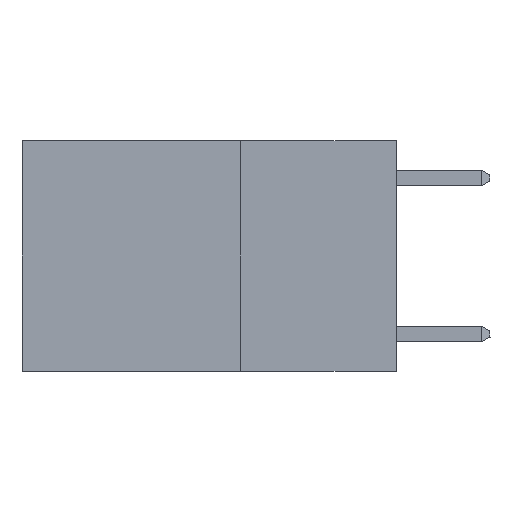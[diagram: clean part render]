
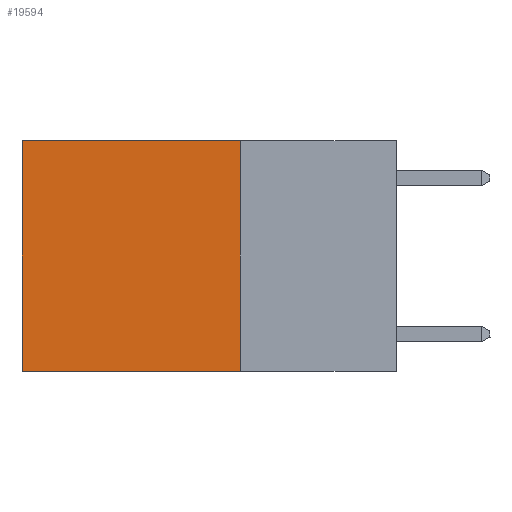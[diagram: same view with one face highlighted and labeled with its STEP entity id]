
A CAD part, left-side view. The second image highlights one B-rep face of the part: STEP entity #19594.
In plain terms, the highlighted planar face has unit normal (-1, 0, 0).
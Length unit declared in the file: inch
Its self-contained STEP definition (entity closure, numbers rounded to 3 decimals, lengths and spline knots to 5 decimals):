
#180 = LINE ( 'NONE', #2613, #320 ) ;
#320 = VECTOR ( 'NONE', #13146, 39.37008 ) ;
#630 = VECTOR ( 'NONE', #18953, 39.37008 ) ;
#824 = LINE ( 'NONE', #12103, #630 ) ;
#914 = ORIENTED_EDGE ( 'NONE', *, *, #18890, .T. ) ;
#1774 = DIRECTION ( 'NONE',  ( 0., 0., -1. ) ) ;
#2613 = CARTESIAN_POINT ( 'NONE',  ( 0.2625, 0.25, 0. ) ) ;
#7074 = CARTESIAN_POINT ( 'NONE',  ( 0.2625, 0.6, 0. ) ) ;
#7731 = EDGE_LOOP ( 'NONE', ( #914, #15957, #12379, #12878 ) ) ;
#8198 = LINE ( 'NONE', #22268, #21597 ) ;
#8571 = CARTESIAN_POINT ( 'NONE',  ( 0.2625, 0.6, 0. ) ) ;
#8824 = DIRECTION ( 'NONE',  ( 0., 0., -1. ) ) ;
#8877 = CARTESIAN_POINT ( 'NONE',  ( 0.2625, 0.25, 0. ) ) ;
#9751 = EDGE_CURVE ( 'NONE', #20449, #17550, #824, .T. ) ;
#10504 = VECTOR ( 'NONE', #8824, 39.37008 ) ;
#10688 = EDGE_CURVE ( 'NONE', #13894, #20034, #180, .T. ) ;
#11238 = CARTESIAN_POINT ( 'NONE',  ( 0.2625, 0.25, 0. ) ) ;
#11998 = CARTESIAN_POINT ( 'NONE',  ( 0.2625, 0.6, -0.37 ) ) ;
#12103 = CARTESIAN_POINT ( 'NONE',  ( 0.2625, 0.25, -0.37 ) ) ;
#12379 = ORIENTED_EDGE ( 'NONE', *, *, #21950, .F. ) ;
#12384 = DIRECTION ( 'NONE',  ( 1., 0., 0. ) ) ;
#12878 = ORIENTED_EDGE ( 'NONE', *, *, #10688, .T. ) ;
#13146 = DIRECTION ( 'NONE',  ( 0., 1., 0. ) ) ;
#13894 = VERTEX_POINT ( 'NONE', #11238 ) ;
#14659 = AXIS2_PLACEMENT_3D ( 'NONE', #8877, #12384, #1774 ) ;
#15957 = ORIENTED_EDGE ( 'NONE', *, *, #9751, .F. ) ;
#17550 = VERTEX_POINT ( 'NONE', #11998 ) ;
#17696 = FACE_OUTER_BOUND ( 'NONE', #7731, .T. ) ;
#18541 = CARTESIAN_POINT ( 'NONE',  ( 0.2625, 0.25, -0.37 ) ) ;
#18890 = EDGE_CURVE ( 'NONE', #20034, #17550, #19016, .T. ) ;
#18953 = DIRECTION ( 'NONE',  ( 0., 1., 0. ) ) ;
#19016 = LINE ( 'NONE', #7074, #10504 ) ;
#19049 = DIRECTION ( 'NONE',  ( 0., 0., -1. ) ) ;
#19594 = ADVANCED_FACE ( 'NONE', ( #17696 ), #22348, .F. ) ;
#20034 = VERTEX_POINT ( 'NONE', #8571 ) ;
#20449 = VERTEX_POINT ( 'NONE', #18541 ) ;
#21597 = VECTOR ( 'NONE', #19049, 39.37008 ) ;
#21950 = EDGE_CURVE ( 'NONE', #13894, #20449, #8198, .T. ) ;
#22268 = CARTESIAN_POINT ( 'NONE',  ( 0.2625, 0.25, 0. ) ) ;
#22348 = PLANE ( 'NONE',  #14659 ) ;
